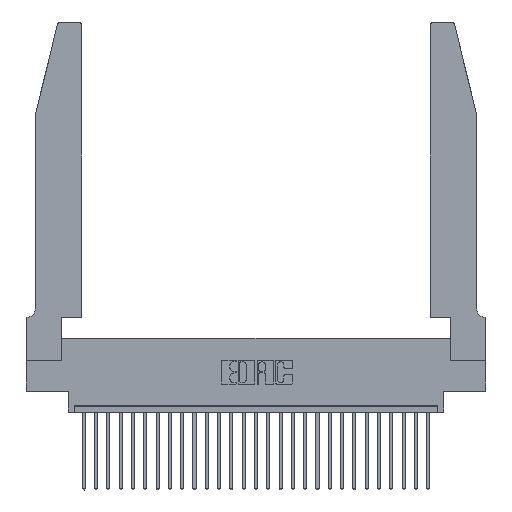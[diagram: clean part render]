
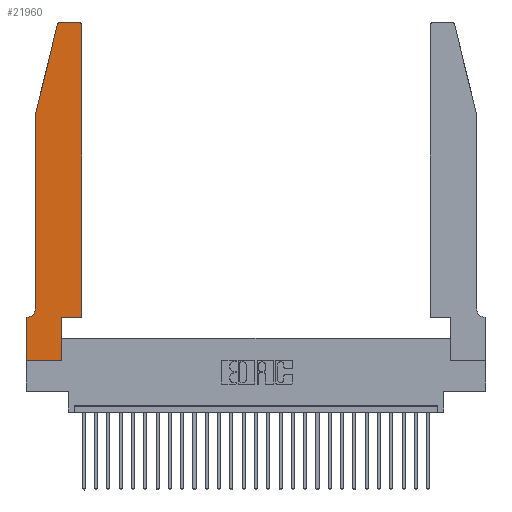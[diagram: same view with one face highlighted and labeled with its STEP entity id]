
A CAD part, top view. The second image highlights one B-rep face of the part: STEP entity #21960.
In plain terms, the highlighted planar face has unit normal (0, 0, 1).
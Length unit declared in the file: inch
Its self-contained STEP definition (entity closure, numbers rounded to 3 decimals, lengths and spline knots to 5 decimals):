
#70 = LINE ( 'NONE', #26680, #13761 ) ;
#120 = FACE_OUTER_BOUND ( 'NONE', #1212, .T. ) ;
#1103 = CARTESIAN_POINT ( 'NONE',  ( 0.0755, 0.35, 0.37 ) ) ;
#1212 = EDGE_LOOP ( 'NONE', ( #2979, #4532, #10916, #7286, #22398, #24654, #16311, #11541, #17764, #2464, #15394, #7656 ) ) ;
#1655 = AXIS2_PLACEMENT_3D ( 'NONE', #16945, #4185, #6081 ) ;
#2130 = EDGE_CURVE ( 'NONE', #28381, #2803, #22353, .T. ) ;
#2138 = DIRECTION ( 'NONE',  ( 1., 0., 0. ) ) ;
#2464 = ORIENTED_EDGE ( 'NONE', *, *, #21580, .T. ) ;
#2803 = VERTEX_POINT ( 'NONE', #17660 ) ;
#2827 = LINE ( 'NONE', #24437, #7250 ) ;
#2979 = ORIENTED_EDGE ( 'NONE', *, *, #18769, .T. ) ;
#3179 = DIRECTION ( 'NONE',  ( 0., 1., 0. ) ) ;
#4030 = DIRECTION ( 'NONE',  ( 0., 0., -1. ) ) ;
#4185 = DIRECTION ( 'NONE',  ( 0., 0., 1. ) ) ;
#4377 = VECTOR ( 'NONE', #28281, 39.37008 ) ;
#4387 = VECTOR ( 'NONE', #4929, 39.37008 ) ;
#4532 = ORIENTED_EDGE ( 'NONE', *, *, #21009, .T. ) ;
#4830 = DIRECTION ( 'NONE',  ( 1., 0., 0. ) ) ;
#4929 = DIRECTION ( 'NONE',  ( 0., 1., 0. ) ) ;
#5291 = VERTEX_POINT ( 'NONE', #18686 ) ;
#5320 = VERTEX_POINT ( 'NONE', #14641 ) ;
#5720 = EDGE_CURVE ( 'NONE', #16224, #13251, #2827, .T. ) ;
#5825 = CARTESIAN_POINT ( 'NONE',  ( 0.284, 2.75, 0.37 ) ) ;
#5936 = CARTESIAN_POINT ( 'NONE',  ( 0.2865, 0., 0.37 ) ) ;
#6081 = DIRECTION ( 'NONE',  ( 1., 0., 0. ) ) ;
#7250 = VECTOR ( 'NONE', #11253, 39.37008 ) ;
#7286 = ORIENTED_EDGE ( 'NONE', *, *, #5720, .T. ) ;
#7656 = ORIENTED_EDGE ( 'NONE', *, *, #19709, .T. ) ;
#7981 = EDGE_CURVE ( 'NONE', #5291, #28381, #11493, .T. ) ;
#9340 = DIRECTION ( 'NONE',  ( 0., 0., 1. ) ) ;
#9363 = AXIS2_PLACEMENT_3D ( 'NONE', #12563, #4030, #19377 ) ;
#9941 = DIRECTION ( 'NONE',  ( 0., -1., 0. ) ) ;
#10140 = VECTOR ( 'NONE', #17797, 39.37008 ) ;
#10568 = VECTOR ( 'NONE', #25628, 39.37008 ) ;
#10916 = ORIENTED_EDGE ( 'NONE', *, *, #15338, .T. ) ;
#11253 = DIRECTION ( 'NONE',  ( 0., -1., 0. ) ) ;
#11337 = CARTESIAN_POINT ( 'NONE',  ( 0.0755, 0.42, 0.37 ) ) ;
#11493 = LINE ( 'NONE', #15163, #28009 ) ;
#11541 = ORIENTED_EDGE ( 'NONE', *, *, #7981, .T. ) ;
#11591 = AXIS2_PLACEMENT_3D ( 'NONE', #28129, #23816, #4830 ) ;
#11659 = EDGE_CURVE ( 'NONE', #13251, #28008, #13040, .T. ) ;
#12563 = CARTESIAN_POINT ( 'NONE',  ( 0.0055, 0.42, 0.37 ) ) ;
#12806 = VECTOR ( 'NONE', #20540, 39.37008 ) ;
#12851 = CARTESIAN_POINT ( 'NONE',  ( 0.0755, 2., 0.37 ) ) ;
#13040 = CIRCLE ( 'NONE', #9363, 0.07 ) ;
#13251 = VERTEX_POINT ( 'NONE', #11337 ) ;
#13347 = EDGE_CURVE ( 'NONE', #25063, #5320, #18383, .T. ) ;
#13663 = CARTESIAN_POINT ( 'NONE',  ( 0.2605, 2.75, 0.37 ) ) ;
#13750 = CARTESIAN_POINT ( 'NONE',  ( 0.2865, 0.35, 0.37 ) ) ;
#13761 = VECTOR ( 'NONE', #9941, 39.37008 ) ;
#13890 = CARTESIAN_POINT ( 'NONE',  ( 0.4205, 2.75, 0.37 ) ) ;
#13893 = LINE ( 'NONE', #13663, #10140 ) ;
#13900 = CARTESIAN_POINT ( 'NONE',  ( 0.25487, 2.72718, 0.37 ) ) ;
#14236 = VECTOR ( 'NONE', #3179, 39.37008 ) ;
#14641 = CARTESIAN_POINT ( 'NONE',  ( 0.4505, 2.72, 0.37 ) ) ;
#15154 = CARTESIAN_POINT ( 'NONE',  ( 0., 0.35, 0.37 ) ) ;
#15163 = CARTESIAN_POINT ( 'NONE',  ( 0., 0., 0.37 ) ) ;
#15294 = CARTESIAN_POINT ( 'NONE',  ( 0.0055, 0.35, 0.37 ) ) ;
#15309 = VERTEX_POINT ( 'NONE', #15154 ) ;
#15338 = EDGE_CURVE ( 'NONE', #16039, #16224, #18800, .T. ) ;
#15394 = ORIENTED_EDGE ( 'NONE', *, *, #13347, .T. ) ;
#15876 = PLANE ( 'NONE',  #21196 ) ;
#16039 = VERTEX_POINT ( 'NONE', #13900 ) ;
#16071 = VERTEX_POINT ( 'NONE', #5825 ) ;
#16209 = CARTESIAN_POINT ( 'NONE',  ( 0.4505, 0.35, 0.37 ) ) ;
#16224 = VERTEX_POINT ( 'NONE', #20159 ) ;
#16311 = ORIENTED_EDGE ( 'NONE', *, *, #22484, .T. ) ;
#16945 = CARTESIAN_POINT ( 'NONE',  ( 0.284, 2.72, 0.37 ) ) ;
#16974 = EDGE_CURVE ( 'NONE', #28008, #15309, #28137, .T. ) ;
#17144 = VERTEX_POINT ( 'NONE', #13890 ) ;
#17306 = CIRCLE ( 'NONE', #1655, 0.03 ) ;
#17660 = CARTESIAN_POINT ( 'NONE',  ( 0.2865, 0.35, 0.37 ) ) ;
#17764 = ORIENTED_EDGE ( 'NONE', *, *, #2130, .T. ) ;
#17797 = DIRECTION ( 'NONE',  ( -1., 0., 0. ) ) ;
#18065 = DIRECTION ( 'NONE',  ( 1., 0., 0. ) ) ;
#18383 = LINE ( 'NONE', #26985, #14236 ) ;
#18686 = CARTESIAN_POINT ( 'NONE',  ( 0., 0., 0.37 ) ) ;
#18769 = EDGE_CURVE ( 'NONE', #17144, #16071, #13893, .T. ) ;
#18800 = LINE ( 'NONE', #12851, #4377 ) ;
#19377 = DIRECTION ( 'NONE',  ( -1., 0., 0. ) ) ;
#19709 = EDGE_CURVE ( 'NONE', #5320, #17144, #26622, .T. ) ;
#20159 = CARTESIAN_POINT ( 'NONE',  ( 0.0755, 2., 0.37 ) ) ;
#20540 = DIRECTION ( 'NONE',  ( 1., 0., 0. ) ) ;
#21009 = EDGE_CURVE ( 'NONE', #16071, #16039, #17306, .T. ) ;
#21196 = AXIS2_PLACEMENT_3D ( 'NONE', #22568, #9340, #18065 ) ;
#21580 = EDGE_CURVE ( 'NONE', #2803, #25063, #24558, .T. ) ;
#21960 = ADVANCED_FACE ( 'NONE', ( #120 ), #15876, .T. ) ;
#22353 = LINE ( 'NONE', #13750, #4387 ) ;
#22398 = ORIENTED_EDGE ( 'NONE', *, *, #11659, .T. ) ;
#22484 = EDGE_CURVE ( 'NONE', #15309, #5291, #70, .T. ) ;
#22568 = CARTESIAN_POINT ( 'NONE',  ( 0., 0.35, 0.37 ) ) ;
#23816 = DIRECTION ( 'NONE',  ( 0., 0., 1. ) ) ;
#23992 = CARTESIAN_POINT ( 'NONE',  ( 0.4505, 0.35, 0.37 ) ) ;
#24437 = CARTESIAN_POINT ( 'NONE',  ( 0.0755, 2., 0.37 ) ) ;
#24558 = LINE ( 'NONE', #16209, #12806 ) ;
#24654 = ORIENTED_EDGE ( 'NONE', *, *, #16974, .T. ) ;
#25063 = VERTEX_POINT ( 'NONE', #23992 ) ;
#25628 = DIRECTION ( 'NONE',  ( -1., 0., 0. ) ) ;
#26622 = CIRCLE ( 'NONE', #11591, 0.03 ) ;
#26680 = CARTESIAN_POINT ( 'NONE',  ( 0., 0., 0.37 ) ) ;
#26985 = CARTESIAN_POINT ( 'NONE',  ( 0.4505, 0.35, 0.37 ) ) ;
#28008 = VERTEX_POINT ( 'NONE', #15294 ) ;
#28009 = VECTOR ( 'NONE', #2138, 39.37008 ) ;
#28129 = CARTESIAN_POINT ( 'NONE',  ( 0.4205, 2.72, 0.37 ) ) ;
#28137 = LINE ( 'NONE', #1103, #10568 ) ;
#28281 = DIRECTION ( 'NONE',  ( -0.239, -0.971, 0. ) ) ;
#28381 = VERTEX_POINT ( 'NONE', #5936 ) ;
